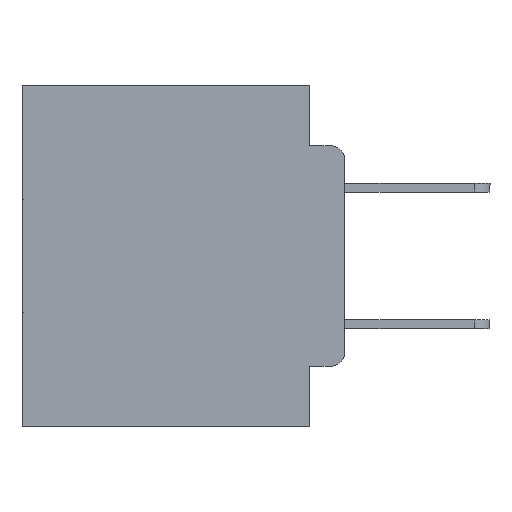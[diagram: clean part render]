
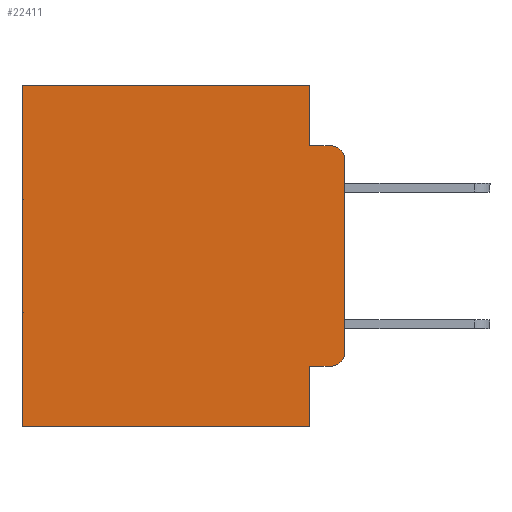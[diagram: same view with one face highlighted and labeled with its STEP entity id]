
A CAD part, left-side view. The second image highlights one B-rep face of the part: STEP entity #22411.
In plain terms, the highlighted planar face has unit normal (-1, 0, 0).
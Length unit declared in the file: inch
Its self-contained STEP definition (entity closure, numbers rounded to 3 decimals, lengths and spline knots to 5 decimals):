
#494 = VECTOR ( 'NONE', #13863, 39.37008 ) ;
#1030 = CARTESIAN_POINT ( 'NONE',  ( 0.298, 0.473, 0. ) ) ;
#1059 = VERTEX_POINT ( 'NONE', #12928 ) ;
#1261 = LINE ( 'NONE', #25622, #494 ) ;
#1648 = ORIENTED_EDGE ( 'NONE', *, *, #16389, .F. ) ;
#1679 = ORIENTED_EDGE ( 'NONE', *, *, #7289, .T. ) ;
#1791 = ORIENTED_EDGE ( 'NONE', *, *, #13255, .F. ) ;
#1922 = VECTOR ( 'NONE', #13559, 39.37008 ) ;
#1954 = LINE ( 'NONE', #3146, #7624 ) ;
#2041 = ORIENTED_EDGE ( 'NONE', *, *, #12400, .F. ) ;
#2403 = ORIENTED_EDGE ( 'NONE', *, *, #18041, .T. ) ;
#2522 = VERTEX_POINT ( 'NONE', #19276 ) ;
#2724 = ORIENTED_EDGE ( 'NONE', *, *, #5882, .T. ) ;
#2755 = DIRECTION ( 'NONE',  ( 0., 1., 0. ) ) ;
#2980 = ORIENTED_EDGE ( 'NONE', *, *, #3651, .F. ) ;
#3146 = CARTESIAN_POINT ( 'NONE',  ( 0.298, 0.051, -0.0885 ) ) ;
#3156 = ORIENTED_EDGE ( 'NONE', *, *, #16604, .F. ) ;
#3417 = ORIENTED_EDGE ( 'NONE', *, *, #13714, .T. ) ;
#3432 = VERTEX_POINT ( 'NONE', #16825 ) ;
#3651 = EDGE_CURVE ( 'NONE', #13335, #3432, #16249, .T. ) ;
#3653 = ORIENTED_EDGE ( 'NONE', *, *, #24029, .T. ) ;
#5046 = CARTESIAN_POINT ( 'NONE',  ( 0.298, 0.051, -0.4115 ) ) ;
#5882 = EDGE_CURVE ( 'NONE', #27828, #3432, #26487, .T. ) ;
#5905 = VERTEX_POINT ( 'NONE', #12773 ) ;
#6414 = VERTEX_POINT ( 'NONE', #10329 ) ;
#7289 = EDGE_CURVE ( 'NONE', #14538, #19484, #26034, .T. ) ;
#7624 = VECTOR ( 'NONE', #17255, 39.37008 ) ;
#8323 = EDGE_LOOP ( 'NONE', ( #1648, #1679, #1791, #2041, #2403, #2724, #2980, #3156, #3417, #3653 ) ) ;
#8797 = DIRECTION ( 'NONE',  ( -1., 0., 0. ) ) ;
#9993 = VECTOR ( 'NONE', #2755, 39.37008 ) ;
#10329 = CARTESIAN_POINT ( 'NONE',  ( 0.298, 0.051, 0. ) ) ;
#10637 = CARTESIAN_POINT ( 'NONE',  ( 0.298, 0.02, -0.3915 ) ) ;
#11643 = DIRECTION ( 'NONE',  ( 1., 0., 0. ) ) ;
#12025 = AXIS2_PLACEMENT_3D ( 'NONE', #13913, #11643, #28099 ) ;
#12400 = EDGE_CURVE ( 'NONE', #6414, #2522, #1261, .T. ) ;
#12773 = CARTESIAN_POINT ( 'NONE',  ( 0.298, 0., -0.3915 ) ) ;
#12928 = CARTESIAN_POINT ( 'NONE',  ( 0.298, 0.02, -0.4115 ) ) ;
#12959 = DIRECTION ( 'NONE',  ( 0., 0., -1. ) ) ;
#13255 = EDGE_CURVE ( 'NONE', #2522, #19484, #1954, .T. ) ;
#13335 = VERTEX_POINT ( 'NONE', #29226 ) ;
#13559 = DIRECTION ( 'NONE',  ( 0., -1., 0. ) ) ;
#13714 = EDGE_CURVE ( 'NONE', #28741, #1059, #15217, .T. ) ;
#13863 = DIRECTION ( 'NONE',  ( 0., 0., -1. ) ) ;
#13897 = FACE_OUTER_BOUND ( 'NONE', #8323, .T. ) ;
#13913 = CARTESIAN_POINT ( 'NONE',  ( 0.298, 0., 0. ) ) ;
#14392 = AXIS2_PLACEMENT_3D ( 'NONE', #22880, #8797, #25203 ) ;
#14538 = VERTEX_POINT ( 'NONE', #26116 ) ;
#15217 = LINE ( 'NONE', #29996, #1922 ) ;
#15789 = LINE ( 'NONE', #21674, #27567 ) ;
#16249 = LINE ( 'NONE', #27168, #9993 ) ;
#16310 = PLANE ( 'NONE',  #12025 ) ;
#16389 = EDGE_CURVE ( 'NONE', #14538, #5905, #15789, .T. ) ;
#16604 = EDGE_CURVE ( 'NONE', #28741, #13335, #16889, .T. ) ;
#16825 = CARTESIAN_POINT ( 'NONE',  ( 0.298, 0.473, -0.5 ) ) ;
#16889 = LINE ( 'NONE', #20105, #28614 ) ;
#17255 = DIRECTION ( 'NONE',  ( 0., -1., 0. ) ) ;
#17562 = DIRECTION ( 'NONE',  ( 0., 0., -1. ) ) ;
#18039 = CARTESIAN_POINT ( 'NONE',  ( 0.298, 0., 0. ) ) ;
#18041 = EDGE_CURVE ( 'NONE', #6414, #27828, #28842, .T. ) ;
#19276 = CARTESIAN_POINT ( 'NONE',  ( 0.298, 0.051, -0.0885 ) ) ;
#19484 = VERTEX_POINT ( 'NONE', #23112 ) ;
#20105 = CARTESIAN_POINT ( 'NONE',  ( 0.298, 0.051, 0. ) ) ;
#20956 = VECTOR ( 'NONE', #17562, 39.37008 ) ;
#21674 = CARTESIAN_POINT ( 'NONE',  ( 0.298, 0., 0. ) ) ;
#21800 = AXIS2_PLACEMENT_3D ( 'NONE', #10637, #27128, #12959 ) ;
#22411 = ADVANCED_FACE ( 'NONE', ( #13897 ), #16310, .F. ) ;
#22486 = DIRECTION ( 'NONE',  ( 0., 0., -1. ) ) ;
#22677 = VECTOR ( 'NONE', #29800, 39.37008 ) ;
#22880 = CARTESIAN_POINT ( 'NONE',  ( 0.298, 0.02, -0.1085 ) ) ;
#23112 = CARTESIAN_POINT ( 'NONE',  ( 0.298, 0.02, -0.0885 ) ) ;
#24029 = EDGE_CURVE ( 'NONE', #1059, #5905, #29950, .T. ) ;
#24037 = DIRECTION ( 'NONE',  ( 0., 0., -1. ) ) ;
#25203 = DIRECTION ( 'NONE',  ( 0., 0., -1. ) ) ;
#25622 = CARTESIAN_POINT ( 'NONE',  ( 0.298, 0.051, 0. ) ) ;
#26034 = CIRCLE ( 'NONE', #14392, 0.02 ) ;
#26116 = CARTESIAN_POINT ( 'NONE',  ( 0.298, 0., -0.1085 ) ) ;
#26487 = LINE ( 'NONE', #1030, #20956 ) ;
#27128 = DIRECTION ( 'NONE',  ( -1., 0., 0. ) ) ;
#27168 = CARTESIAN_POINT ( 'NONE',  ( 0.298, 0., -0.5 ) ) ;
#27567 = VECTOR ( 'NONE', #24037, 39.37008 ) ;
#27828 = VERTEX_POINT ( 'NONE', #28064 ) ;
#28064 = CARTESIAN_POINT ( 'NONE',  ( 0.298, 0.473, 0. ) ) ;
#28099 = DIRECTION ( 'NONE',  ( 0., 0., -1. ) ) ;
#28614 = VECTOR ( 'NONE', #22486, 39.37008 ) ;
#28741 = VERTEX_POINT ( 'NONE', #5046 ) ;
#28842 = LINE ( 'NONE', #18039, #22677 ) ;
#29226 = CARTESIAN_POINT ( 'NONE',  ( 0.298, 0.051, -0.5 ) ) ;
#29800 = DIRECTION ( 'NONE',  ( 0., 1., 0. ) ) ;
#29950 = CIRCLE ( 'NONE', #21800, 0.02 ) ;
#29996 = CARTESIAN_POINT ( 'NONE',  ( 0.298, 0.051, -0.4115 ) ) ;
